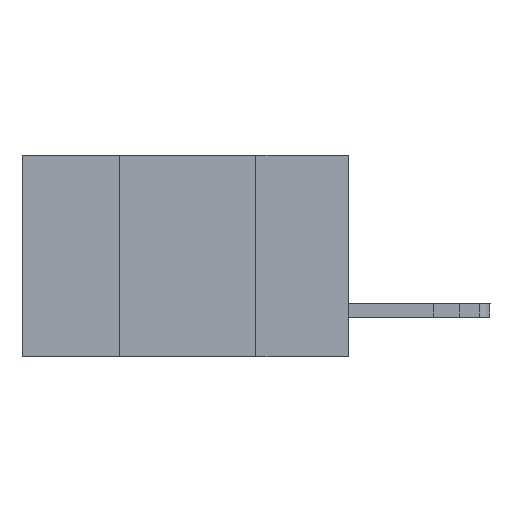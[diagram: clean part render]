
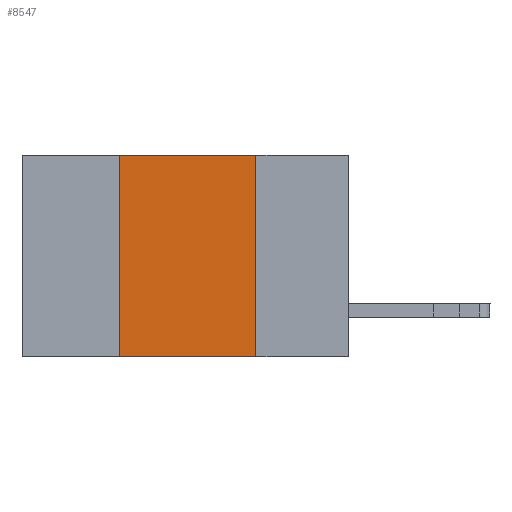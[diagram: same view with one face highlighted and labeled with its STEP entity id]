
A CAD part, left-side view. The second image highlights one B-rep face of the part: STEP entity #8547.
In plain terms, the highlighted planar face has unit normal (-1, 0, 0).
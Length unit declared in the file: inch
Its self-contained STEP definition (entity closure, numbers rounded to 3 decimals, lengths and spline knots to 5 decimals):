
#704 = DIRECTION ( 'NONE',  ( 0., 0., -1. ) ) ;
#792 = VERTEX_POINT ( 'NONE', #7128 ) ;
#848 = FACE_OUTER_BOUND ( 'NONE', #8162, .T. ) ;
#1114 = EDGE_CURVE ( 'NONE', #792, #6443, #6813, .T. ) ;
#1275 = CARTESIAN_POINT ( 'NONE',  ( 0., 0.17, -0.37 ) ) ;
#1301 = CARTESIAN_POINT ( 'NONE',  ( 0., 0.42, -0.37 ) ) ;
#1401 = ORIENTED_EDGE ( 'NONE', *, *, #4825, .F. ) ;
#1946 = DIRECTION ( 'NONE',  ( 0., 0., 1. ) ) ;
#2383 = ORIENTED_EDGE ( 'NONE', *, *, #10013, .T. ) ;
#2702 = VERTEX_POINT ( 'NONE', #1301 ) ;
#2828 = DIRECTION ( 'NONE',  ( 0., -1., 0. ) ) ;
#3277 = CARTESIAN_POINT ( 'NONE',  ( 0., 0.17, 0. ) ) ;
#3744 = CARTESIAN_POINT ( 'NONE',  ( 0., 0.42, -0.37 ) ) ;
#4546 = ORIENTED_EDGE ( 'NONE', *, *, #6192, .F. ) ;
#4726 = AXIS2_PLACEMENT_3D ( 'NONE', #8689, #10255, #704 ) ;
#4749 = VECTOR ( 'NONE', #8844, 39.37008 ) ;
#4799 = CARTESIAN_POINT ( 'NONE',  ( 0., 0.17, -0.37 ) ) ;
#4821 = VERTEX_POINT ( 'NONE', #1275 ) ;
#4825 = EDGE_CURVE ( 'NONE', #2702, #792, #8553, .T. ) ;
#6062 = DIRECTION ( 'NONE',  ( 0., -1., 0. ) ) ;
#6076 = CARTESIAN_POINT ( 'NONE',  ( 0., 0.6, -0.37 ) ) ;
#6192 = EDGE_CURVE ( 'NONE', #6443, #4821, #9629, .T. ) ;
#6246 = VECTOR ( 'NONE', #2828, 39.37008 ) ;
#6274 = VECTOR ( 'NONE', #6062, 39.37008 ) ;
#6443 = VERTEX_POINT ( 'NONE', #3277 ) ;
#6813 = LINE ( 'NONE', #9208, #6274 ) ;
#6925 = VECTOR ( 'NONE', #1946, 39.37008 ) ;
#7024 = ORIENTED_EDGE ( 'NONE', *, *, #1114, .F. ) ;
#7128 = CARTESIAN_POINT ( 'NONE',  ( 0., 0.42, 0. ) ) ;
#8162 = EDGE_LOOP ( 'NONE', ( #4546, #7024, #1401, #2383 ) ) ;
#8449 = LINE ( 'NONE', #6076, #6246 ) ;
#8547 = ADVANCED_FACE ( 'NONE', ( #848 ), #10305, .F. ) ;
#8553 = LINE ( 'NONE', #3744, #6925 ) ;
#8689 = CARTESIAN_POINT ( 'NONE',  ( 0., 0.6, 0. ) ) ;
#8844 = DIRECTION ( 'NONE',  ( 0., 0., -1. ) ) ;
#9208 = CARTESIAN_POINT ( 'NONE',  ( 0., 0.6, 0. ) ) ;
#9629 = LINE ( 'NONE', #4799, #4749 ) ;
#10013 = EDGE_CURVE ( 'NONE', #2702, #4821, #8449, .T. ) ;
#10255 = DIRECTION ( 'NONE',  ( 1., 0., 0. ) ) ;
#10305 = PLANE ( 'NONE',  #4726 ) ;
